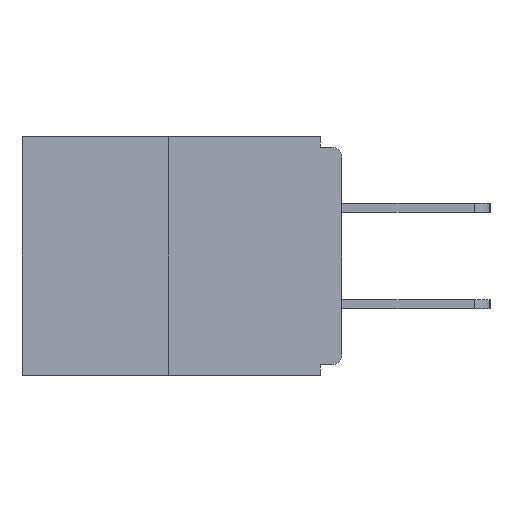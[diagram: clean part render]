
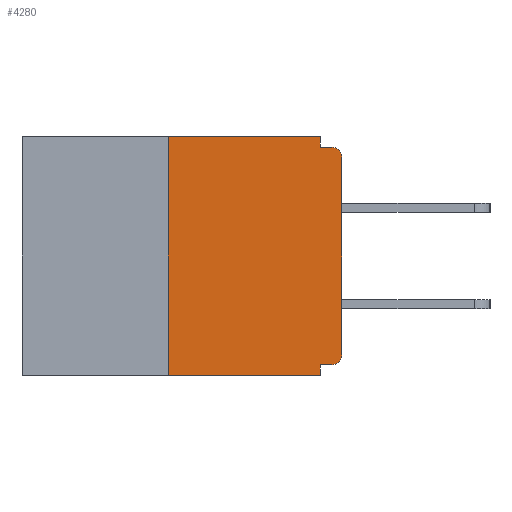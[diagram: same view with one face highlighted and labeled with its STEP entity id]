
A CAD part, left-side view. The second image highlights one B-rep face of the part: STEP entity #4280.
In plain terms, the highlighted planar face has unit normal (-1, 0, 0).
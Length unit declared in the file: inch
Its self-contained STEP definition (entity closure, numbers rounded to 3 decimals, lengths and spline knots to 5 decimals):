
#156 = CARTESIAN_POINT ( 'NONE',  ( 0., 0.031, 0. ) ) ;
#680 = DIRECTION ( 'NONE',  ( 0., -1., 0. ) ) ;
#749 = EDGE_CURVE ( 'NONE', #5841, #4166, #10409, .T. ) ;
#1029 = EDGE_CURVE ( 'NONE', #3023, #11526, #11632, .T. ) ;
#1193 = CARTESIAN_POINT ( 'NONE',  ( 0., 0., -0.313 ) ) ;
#1377 = ORIENTED_EDGE ( 'NONE', *, *, #1029, .T. ) ;
#1495 = DIRECTION ( 'NONE',  ( 0., 1., 0. ) ) ;
#1641 = ORIENTED_EDGE ( 'NONE', *, *, #2575, .F. ) ;
#1909 = CARTESIAN_POINT ( 'NONE',  ( 0., 0., -0.015 ) ) ;
#1924 = EDGE_CURVE ( 'NONE', #4166, #8561, #15848, .T. ) ;
#2010 = AXIS2_PLACEMENT_3D ( 'NONE', #15430, #16412, #11242 ) ;
#2022 = CARTESIAN_POINT ( 'NONE',  ( 0., 0.031, 0. ) ) ;
#2575 = EDGE_CURVE ( 'NONE', #3215, #4351, #11772, .T. ) ;
#2628 = VERTEX_POINT ( 'NONE', #156 ) ;
#2754 = CARTESIAN_POINT ( 'NONE',  ( 0., 0.46, 0. ) ) ;
#2825 = AXIS2_PLACEMENT_3D ( 'NONE', #6886, #4390, #10741 ) ;
#2919 = VECTOR ( 'NONE', #6582, 39.37008 ) ;
#3023 = VERTEX_POINT ( 'NONE', #12496 ) ;
#3197 = CARTESIAN_POINT ( 'NONE',  ( 0., 0.031, -0.343 ) ) ;
#3215 = VERTEX_POINT ( 'NONE', #12942 ) ;
#3516 = EDGE_CURVE ( 'NONE', #4351, #2628, #10318, .T. ) ;
#4019 = CARTESIAN_POINT ( 'NONE',  ( 0., 0.46, -0.343 ) ) ;
#4166 = VERTEX_POINT ( 'NONE', #9576 ) ;
#4280 = ADVANCED_FACE ( 'NONE', ( #9256 ), #15093, .F. ) ;
#4286 = VECTOR ( 'NONE', #11783, 39.37008 ) ;
#4351 = VERTEX_POINT ( 'NONE', #9980 ) ;
#4390 = DIRECTION ( 'NONE',  ( -1., 0., 0. ) ) ;
#4721 = CARTESIAN_POINT ( 'NONE',  ( 0., 0.015, -0.03 ) ) ;
#4748 = ORIENTED_EDGE ( 'NONE', *, *, #12497, .F. ) ;
#5253 = CARTESIAN_POINT ( 'NONE',  ( 0., 0.015, -0.015 ) ) ;
#5487 = LINE ( 'NONE', #11003, #11930 ) ;
#5834 = CARTESIAN_POINT ( 'NONE',  ( 0., 0.031, -0.015 ) ) ;
#5841 = VERTEX_POINT ( 'NONE', #8440 ) ;
#5874 = EDGE_CURVE ( 'NONE', #2628, #15856, #12666, .T. ) ;
#6345 = VECTOR ( 'NONE', #11103, 39.37008 ) ;
#6571 = ORIENTED_EDGE ( 'NONE', *, *, #15909, .T. ) ;
#6582 = DIRECTION ( 'NONE',  ( 0., -1., 0. ) ) ;
#6886 = CARTESIAN_POINT ( 'NONE',  ( 0., 0.015, -0.313 ) ) ;
#6927 = EDGE_LOOP ( 'NONE', ( #15719, #1641, #14829, #13209, #12200, #8758, #6571, #1377, #4748, #12851 ) ) ;
#7049 = DIRECTION ( 'NONE',  ( 0., 0., 1. ) ) ;
#7574 = AXIS2_PLACEMENT_3D ( 'NONE', #4721, #15157, #14925 ) ;
#7973 = VERTEX_POINT ( 'NONE', #1193 ) ;
#8440 = CARTESIAN_POINT ( 'NONE',  ( 0., 0.015, -0.328 ) ) ;
#8498 = DIRECTION ( 'NONE',  ( 0., 0., -1. ) ) ;
#8535 = VECTOR ( 'NONE', #8877, 39.37008 ) ;
#8561 = VERTEX_POINT ( 'NONE', #3197 ) ;
#8758 = ORIENTED_EDGE ( 'NONE', *, *, #13347, .T. ) ;
#8877 = DIRECTION ( 'NONE',  ( 0., 0., 1. ) ) ;
#9193 = CARTESIAN_POINT ( 'NONE',  ( 0., 0., -0.328 ) ) ;
#9256 = FACE_OUTER_BOUND ( 'NONE', #6927, .T. ) ;
#9576 = CARTESIAN_POINT ( 'NONE',  ( 0., 0.031, -0.328 ) ) ;
#9980 = CARTESIAN_POINT ( 'NONE',  ( 0., 0.25, 0. ) ) ;
#9997 = EDGE_CURVE ( 'NONE', #3215, #8561, #14848, .T. ) ;
#10318 = LINE ( 'NONE', #2754, #4286 ) ;
#10409 = LINE ( 'NONE', #9193, #13667 ) ;
#10741 = DIRECTION ( 'NONE',  ( 0., 0., -1. ) ) ;
#11003 = CARTESIAN_POINT ( 'NONE',  ( 0., 0., 0. ) ) ;
#11103 = DIRECTION ( 'NONE',  ( 0., 0., -1. ) ) ;
#11242 = DIRECTION ( 'NONE',  ( 0., 0., -1. ) ) ;
#11526 = VERTEX_POINT ( 'NONE', #5253 ) ;
#11632 = CIRCLE ( 'NONE', #7574, 0.015 ) ;
#11660 = VECTOR ( 'NONE', #8498, 39.37008 ) ;
#11772 = LINE ( 'NONE', #16668, #8535 ) ;
#11783 = DIRECTION ( 'NONE',  ( 0., -1., 0. ) ) ;
#11930 = VECTOR ( 'NONE', #7049, 39.37008 ) ;
#12200 = ORIENTED_EDGE ( 'NONE', *, *, #749, .F. ) ;
#12496 = CARTESIAN_POINT ( 'NONE',  ( 0., 0., -0.03 ) ) ;
#12497 = EDGE_CURVE ( 'NONE', #15856, #11526, #14174, .T. ) ;
#12666 = LINE ( 'NONE', #2022, #11660 ) ;
#12851 = ORIENTED_EDGE ( 'NONE', *, *, #5874, .F. ) ;
#12942 = CARTESIAN_POINT ( 'NONE',  ( 0., 0.25, -0.343 ) ) ;
#13209 = ORIENTED_EDGE ( 'NONE', *, *, #1924, .F. ) ;
#13347 = EDGE_CURVE ( 'NONE', #5841, #7973, #14714, .T. ) ;
#13667 = VECTOR ( 'NONE', #1495, 39.37008 ) ;
#13725 = CARTESIAN_POINT ( 'NONE',  ( 0., 0.031, -0.343 ) ) ;
#14174 = LINE ( 'NONE', #1909, #14966 ) ;
#14714 = CIRCLE ( 'NONE', #2825, 0.015 ) ;
#14829 = ORIENTED_EDGE ( 'NONE', *, *, #9997, .T. ) ;
#14848 = LINE ( 'NONE', #4019, #2919 ) ;
#14925 = DIRECTION ( 'NONE',  ( 0., 0., -1. ) ) ;
#14966 = VECTOR ( 'NONE', #680, 39.37008 ) ;
#15093 = PLANE ( 'NONE',  #2010 ) ;
#15157 = DIRECTION ( 'NONE',  ( -1., 0., 0. ) ) ;
#15430 = CARTESIAN_POINT ( 'NONE',  ( 0., 0.46, 0. ) ) ;
#15719 = ORIENTED_EDGE ( 'NONE', *, *, #3516, .F. ) ;
#15848 = LINE ( 'NONE', #13725, #6345 ) ;
#15856 = VERTEX_POINT ( 'NONE', #5834 ) ;
#15909 = EDGE_CURVE ( 'NONE', #7973, #3023, #5487, .T. ) ;
#16412 = DIRECTION ( 'NONE',  ( 1., 0., 0. ) ) ;
#16668 = CARTESIAN_POINT ( 'NONE',  ( 0., 0.25, 0. ) ) ;
